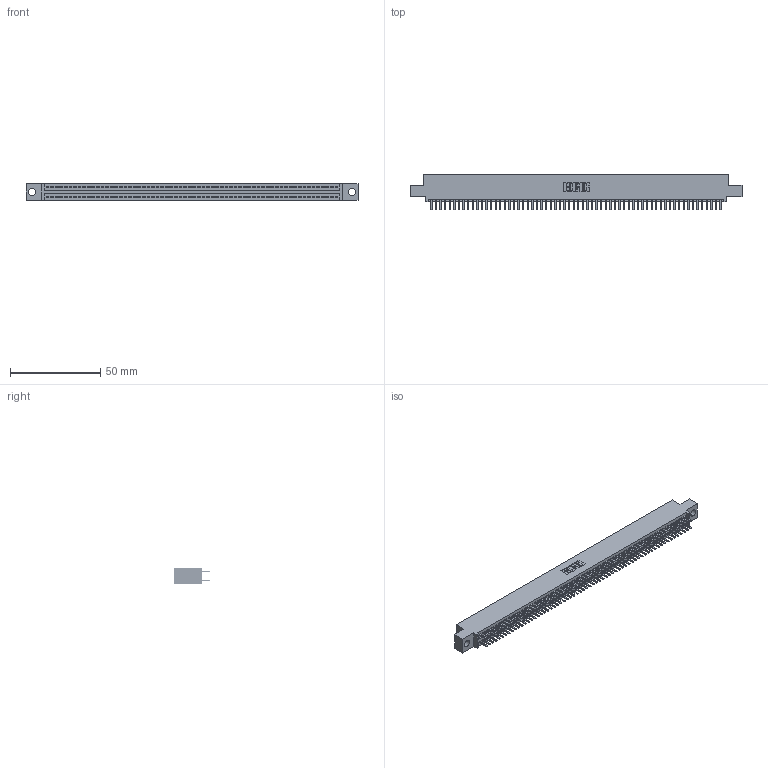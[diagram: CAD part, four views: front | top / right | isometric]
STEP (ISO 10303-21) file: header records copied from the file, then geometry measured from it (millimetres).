
FILE_DESCRIPTION (( 'STEP AP203' ), '1' );
FILE_NAME ('395-128-520-504.STEP', '2018-12-04T09:24:12', ( '' ), ( '' ), 'SwSTEP 2.0', 'SolidWorks 2016', '' );
FILE_SCHEMA (( 'CONFIG_CONTROL_DESIGN' ));
Length unit declared in the file: inch
Products named in the file (3): 395-128-520-504; 345-292-001_345-293-120; 345 Part_0.110 Offset - 0.156 Dia-TH
Assembly tree (129 placements, depth 2):
  395-128-520-504
    345 Part_0.110 Offset - 0.156 Dia-TH
    345-292-001_345-293-120  x128
Bounding box: 183.77 x 19.68 x 9.4 mm (x, y, z)
Volume: 17838.2 mm3; surface area: 26582.3 mm2
Topology: 129 solids, 129 shells, 7042 faces, 20449 edges, 13290 vertices
Faces by surface type: plane 4564, cylinder 2478
Entity records: 47503 total; most frequent: CARTESIAN_POINT 7956, ORIENTED_EDGE 7878, DIRECTION 6975, EDGE_CURVE 3939, VECTOR 3547, LINE 3547, VERTEX_POINT 2622, AXIS2_PLACEMENT_3D 1714
